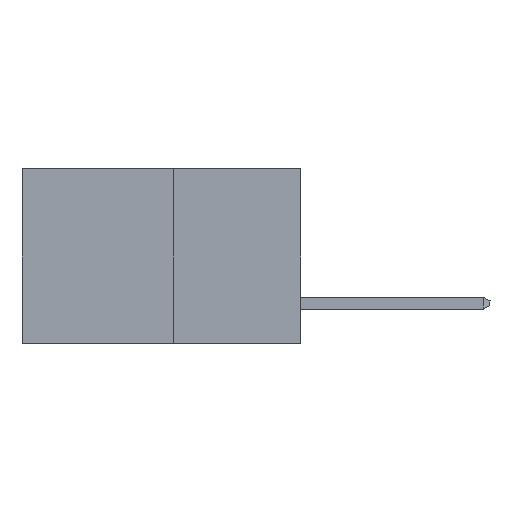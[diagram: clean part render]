
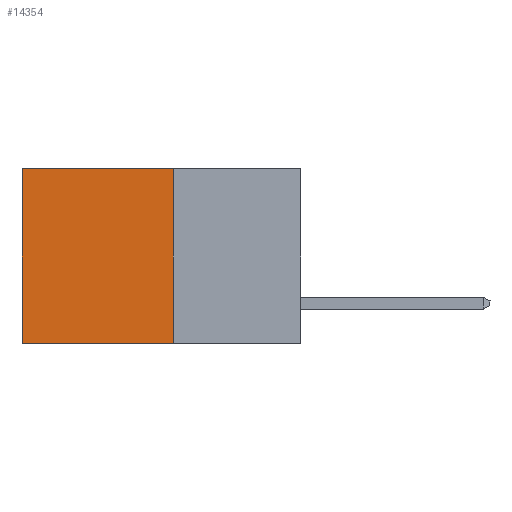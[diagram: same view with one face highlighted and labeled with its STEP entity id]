
A CAD part, left-side view. The second image highlights one B-rep face of the part: STEP entity #14354.
In plain terms, the highlighted planar face has unit normal (-1, 0, 0).
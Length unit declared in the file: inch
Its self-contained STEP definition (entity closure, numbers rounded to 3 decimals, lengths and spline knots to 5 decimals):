
#1973 = CARTESIAN_POINT ( 'NONE',  ( 0.277, 0.27, -0.37 ) ) ;
#2435 = VECTOR ( 'NONE', #10522, 39.37008 ) ;
#3638 = FACE_OUTER_BOUND ( 'NONE', #21779, .T. ) ;
#3645 = LINE ( 'NONE', #16745, #29461 ) ;
#3829 = VERTEX_POINT ( 'NONE', #17271 ) ;
#6850 = VERTEX_POINT ( 'NONE', #22612 ) ;
#7976 = CARTESIAN_POINT ( 'NONE',  ( 0.277, 0.27, 0. ) ) ;
#8168 = ORIENTED_EDGE ( 'NONE', *, *, #28265, .F. ) ;
#9221 = CARTESIAN_POINT ( 'NONE',  ( 0.277, 0.27, -0.37 ) ) ;
#9626 = PLANE ( 'NONE',  #24192 ) ;
#9748 = LINE ( 'NONE', #9221, #22253 ) ;
#9885 = CARTESIAN_POINT ( 'NONE',  ( 0.277, 0.59, 0. ) ) ;
#10522 = DIRECTION ( 'NONE',  ( 0., 1., 0. ) ) ;
#11322 = VERTEX_POINT ( 'NONE', #9885 ) ;
#11364 = ORIENTED_EDGE ( 'NONE', *, *, #29177, .F. ) ;
#11409 = LINE ( 'NONE', #16093, #30496 ) ;
#11770 = CARTESIAN_POINT ( 'NONE',  ( 0.277, 0.27, -0.37 ) ) ;
#12155 = DIRECTION ( 'NONE',  ( 0., 0., -1. ) ) ;
#12249 = ORIENTED_EDGE ( 'NONE', *, *, #26447, .T. ) ;
#13517 = EDGE_CURVE ( 'NONE', #3829, #11322, #21866, .T. ) ;
#14354 = ADVANCED_FACE ( 'NONE', ( #3638 ), #9626, .F. ) ;
#15464 = VERTEX_POINT ( 'NONE', #11770 ) ;
#16093 = CARTESIAN_POINT ( 'NONE',  ( 0.277, 0.27, -0.37 ) ) ;
#16745 = CARTESIAN_POINT ( 'NONE',  ( 0.277, 0.59, -0.37 ) ) ;
#17271 = CARTESIAN_POINT ( 'NONE',  ( 0.277, 0.27, 0. ) ) ;
#18596 = DIRECTION ( 'NONE',  ( 0., 0., -1. ) ) ;
#21779 = EDGE_LOOP ( 'NONE', ( #12249, #11364, #8168, #23703 ) ) ;
#21866 = LINE ( 'NONE', #7976, #2435 ) ;
#22207 = DIRECTION ( 'NONE',  ( 0., 1., 0. ) ) ;
#22253 = VECTOR ( 'NONE', #22207, 39.37008 ) ;
#22612 = CARTESIAN_POINT ( 'NONE',  ( 0.277, 0.59, -0.37 ) ) ;
#23703 = ORIENTED_EDGE ( 'NONE', *, *, #13517, .T. ) ;
#24192 = AXIS2_PLACEMENT_3D ( 'NONE', #1973, #27054, #12155 ) ;
#24202 = DIRECTION ( 'NONE',  ( 0., 0., -1. ) ) ;
#26447 = EDGE_CURVE ( 'NONE', #11322, #6850, #3645, .T. ) ;
#27054 = DIRECTION ( 'NONE',  ( 1., 0., 0. ) ) ;
#28265 = EDGE_CURVE ( 'NONE', #3829, #15464, #11409, .T. ) ;
#29177 = EDGE_CURVE ( 'NONE', #15464, #6850, #9748, .T. ) ;
#29461 = VECTOR ( 'NONE', #24202, 39.37008 ) ;
#30496 = VECTOR ( 'NONE', #18596, 39.37008 ) ;
